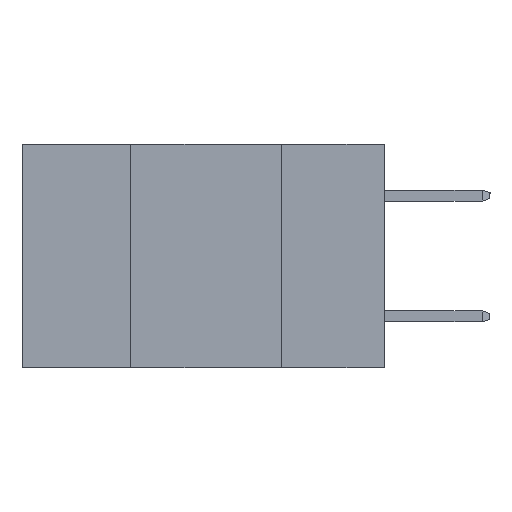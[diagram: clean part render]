
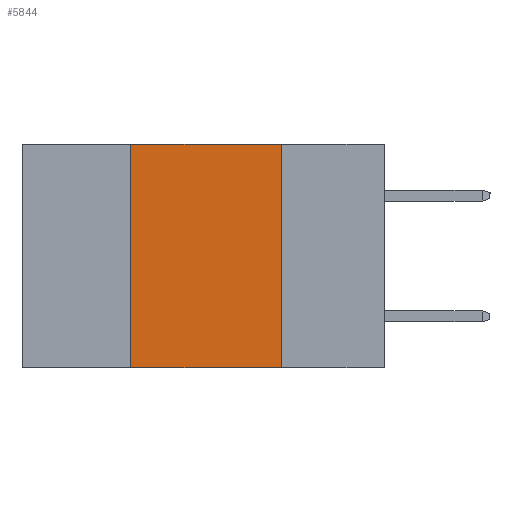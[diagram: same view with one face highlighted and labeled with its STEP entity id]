
A CAD part, left-side view. The second image highlights one B-rep face of the part: STEP entity #5844.
In plain terms, the highlighted planar face has unit normal (-1, 0, 0).
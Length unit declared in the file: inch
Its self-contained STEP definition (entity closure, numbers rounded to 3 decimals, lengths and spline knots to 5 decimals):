
#54 = EDGE_CURVE ( 'NONE', #7406, #195, #409, .T. ) ;
#195 = VERTEX_POINT ( 'NONE', #9986 ) ;
#371 = VECTOR ( 'NONE', #9216, 39.37008 ) ;
#409 = LINE ( 'NONE', #1280, #4421 ) ;
#521 = DIRECTION ( 'NONE',  ( 0., -1., 0. ) ) ;
#530 = CARTESIAN_POINT ( 'NONE',  ( 0., 0.17, -0.37 ) ) ;
#568 = ORIENTED_EDGE ( 'NONE', *, *, #5960, .T. ) ;
#658 = LINE ( 'NONE', #2254, #371 ) ;
#790 = VERTEX_POINT ( 'NONE', #530 ) ;
#1280 = CARTESIAN_POINT ( 'NONE',  ( 0., 0.6, 0. ) ) ;
#1613 = CARTESIAN_POINT ( 'NONE',  ( 0., 0.42, -0.37 ) ) ;
#1713 = AXIS2_PLACEMENT_3D ( 'NONE', #7676, #2072, #8420 ) ;
#1781 = CARTESIAN_POINT ( 'NONE',  ( 0., 0.42, -0.37 ) ) ;
#2017 = FACE_OUTER_BOUND ( 'NONE', #8762, .T. ) ;
#2072 = DIRECTION ( 'NONE',  ( 1., 0., 0. ) ) ;
#2254 = CARTESIAN_POINT ( 'NONE',  ( 0., 0.17, -0.37 ) ) ;
#2995 = ORIENTED_EDGE ( 'NONE', *, *, #54, .F. ) ;
#4421 = VECTOR ( 'NONE', #521, 39.37008 ) ;
#4574 = EDGE_CURVE ( 'NONE', #5217, #7406, #8764, .T. ) ;
#4705 = DIRECTION ( 'NONE',  ( 0., 0., 1. ) ) ;
#5217 = VERTEX_POINT ( 'NONE', #1781 ) ;
#5844 = ADVANCED_FACE ( 'NONE', ( #2017 ), #6075, .F. ) ;
#5960 = EDGE_CURVE ( 'NONE', #5217, #790, #8672, .T. ) ;
#5997 = VECTOR ( 'NONE', #4705, 39.37008 ) ;
#6075 = PLANE ( 'NONE',  #1713 ) ;
#6444 = CARTESIAN_POINT ( 'NONE',  ( 0., 0.42, 0. ) ) ;
#6720 = ORIENTED_EDGE ( 'NONE', *, *, #4574, .F. ) ;
#7406 = VERTEX_POINT ( 'NONE', #6444 ) ;
#7676 = CARTESIAN_POINT ( 'NONE',  ( 0., 0.6, 0. ) ) ;
#7921 = CARTESIAN_POINT ( 'NONE',  ( 0., 0.6, -0.37 ) ) ;
#8205 = EDGE_CURVE ( 'NONE', #195, #790, #658, .T. ) ;
#8420 = DIRECTION ( 'NONE',  ( 0., 0., -1. ) ) ;
#8672 = LINE ( 'NONE', #7921, #9399 ) ;
#8762 = EDGE_LOOP ( 'NONE', ( #10057, #2995, #6720, #568 ) ) ;
#8764 = LINE ( 'NONE', #1613, #5997 ) ;
#9216 = DIRECTION ( 'NONE',  ( 0., 0., -1. ) ) ;
#9399 = VECTOR ( 'NONE', #9744, 39.37008 ) ;
#9744 = DIRECTION ( 'NONE',  ( 0., -1., 0. ) ) ;
#9986 = CARTESIAN_POINT ( 'NONE',  ( 0., 0.17, 0. ) ) ;
#10057 = ORIENTED_EDGE ( 'NONE', *, *, #8205, .F. ) ;
